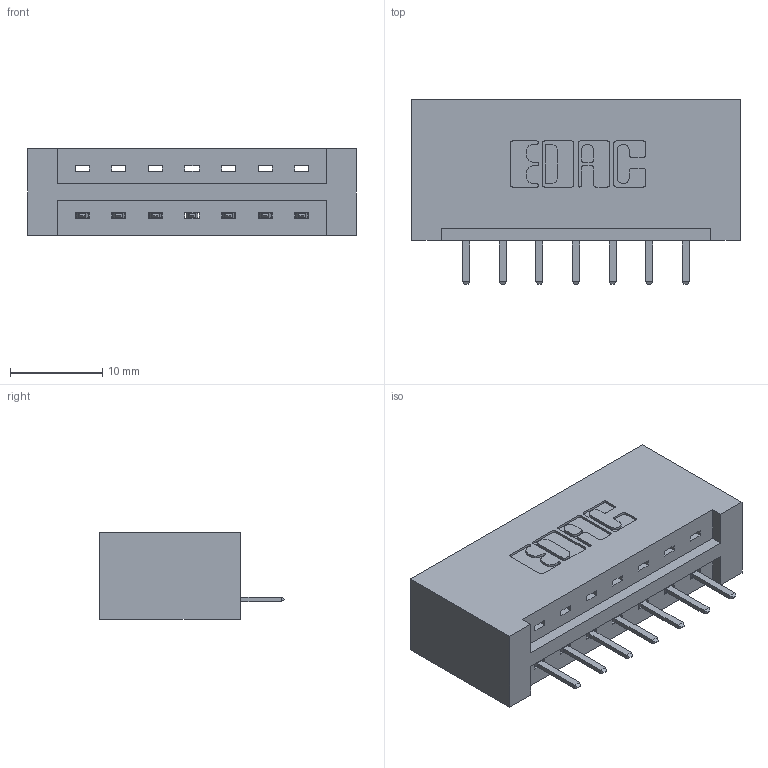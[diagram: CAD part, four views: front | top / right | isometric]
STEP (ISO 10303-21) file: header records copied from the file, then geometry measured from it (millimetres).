
FILE_DESCRIPTION (( 'STEP AP203' ), '1' );
FILE_NAME ('337-007-520-101.STEP', '2019-09-27T17:34:37', ( '' ), ( '' ), 'SwSTEP 2.0', 'SolidWorks 2016', '' );
FILE_SCHEMA (( 'CONFIG_CONTROL_DESIGN' ));
Length unit declared in the file: inch
Products named in the file (3): 345-292-001_345-293-120; 337-007-520-101; 337 Part_No Mounting Lugs
Assembly tree (8 placements, depth 2):
  337-007-520-101
    337 Part_No Mounting Lugs
    345-292-001_345-293-120  x7
Bounding box: 35.61 x 20.02 x 9.4 mm (x, y, z)
Volume: 3981.7 mm3; surface area: 3829.2 mm2
Topology: 8 solids, 8 shells, 568 faces, 1659 edges, 1086 vertices
Faces by surface type: plane 402, cylinder 166
Entity records: 9567 total; most frequent: CARTESIAN_POINT 1683, ORIENTED_EDGE 1614, DIRECTION 1469, EDGE_CURVE 807, LINE 683, VECTOR 683, VERTEX_POINT 534, AXIS2_PLACEMENT_3D 393
